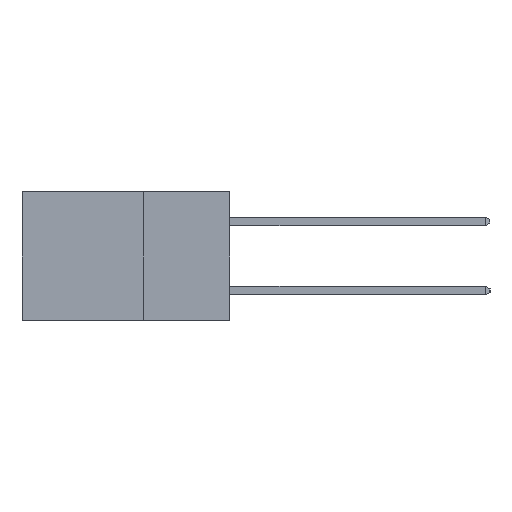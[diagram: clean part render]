
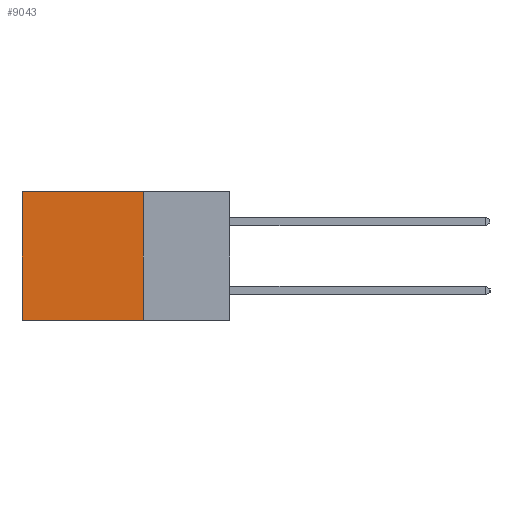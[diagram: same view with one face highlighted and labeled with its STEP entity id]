
A CAD part, left-side view. The second image highlights one B-rep face of the part: STEP entity #9043.
In plain terms, the highlighted planar face has unit normal (-1, 0, 0).
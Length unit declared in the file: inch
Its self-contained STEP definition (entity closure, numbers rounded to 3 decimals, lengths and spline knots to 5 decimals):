
#22 = CARTESIAN_POINT ( 'NONE',  ( 0.2615, 0.25, 0. ) ) ;
#853 = ORIENTED_EDGE ( 'NONE', *, *, #17617, .F. ) ;
#1217 = LINE ( 'NONE', #5633, #9360 ) ;
#1720 = ORIENTED_EDGE ( 'NONE', *, *, #5331, .T. ) ;
#2289 = EDGE_CURVE ( 'NONE', #4972, #5631, #1217, .T. ) ;
#2416 = CARTESIAN_POINT ( 'NONE',  ( 0.2615, 0.25, -0.37 ) ) ;
#2460 = FACE_OUTER_BOUND ( 'NONE', #6613, .T. ) ;
#3838 = VECTOR ( 'NONE', #12416, 39.37008 ) ;
#4061 = DIRECTION ( 'NONE',  ( 0., 0., -1. ) ) ;
#4581 = CARTESIAN_POINT ( 'NONE',  ( 0.2615, 0.6, 0. ) ) ;
#4972 = VERTEX_POINT ( 'NONE', #22 ) ;
#5236 = VERTEX_POINT ( 'NONE', #17708 ) ;
#5331 = EDGE_CURVE ( 'NONE', #5631, #5236, #5470, .T. ) ;
#5470 = LINE ( 'NONE', #16130, #13399 ) ;
#5631 = VERTEX_POINT ( 'NONE', #4581 ) ;
#5633 = CARTESIAN_POINT ( 'NONE',  ( 0.2615, 0.25, 0. ) ) ;
#6613 = EDGE_LOOP ( 'NONE', ( #1720, #853, #10607, #8937 ) ) ;
#7874 = VECTOR ( 'NONE', #10093, 39.37008 ) ;
#8937 = ORIENTED_EDGE ( 'NONE', *, *, #2289, .T. ) ;
#9043 = ADVANCED_FACE ( 'NONE', ( #2460 ), #12059, .F. ) ;
#9360 = VECTOR ( 'NONE', #15056, 39.37008 ) ;
#10093 = DIRECTION ( 'NONE',  ( 0., 1., 0. ) ) ;
#10607 = ORIENTED_EDGE ( 'NONE', *, *, #16162, .F. ) ;
#10828 = CARTESIAN_POINT ( 'NONE',  ( 0.2615, 0.25, -0.37 ) ) ;
#11309 = VERTEX_POINT ( 'NONE', #18542 ) ;
#11582 = CARTESIAN_POINT ( 'NONE',  ( 0.2615, 0.25, -0.37 ) ) ;
#12059 = PLANE ( 'NONE',  #14139 ) ;
#12416 = DIRECTION ( 'NONE',  ( 0., 0., -1. ) ) ;
#13399 = VECTOR ( 'NONE', #16199, 39.37008 ) ;
#13585 = DIRECTION ( 'NONE',  ( 1., 0., 0. ) ) ;
#14139 = AXIS2_PLACEMENT_3D ( 'NONE', #2416, #13585, #4061 ) ;
#15056 = DIRECTION ( 'NONE',  ( 0., 1., 0. ) ) ;
#16130 = CARTESIAN_POINT ( 'NONE',  ( 0.2615, 0.6, -0.37 ) ) ;
#16162 = EDGE_CURVE ( 'NONE', #4972, #11309, #16332, .T. ) ;
#16199 = DIRECTION ( 'NONE',  ( 0., 0., -1. ) ) ;
#16332 = LINE ( 'NONE', #10828, #3838 ) ;
#17617 = EDGE_CURVE ( 'NONE', #11309, #5236, #19938, .T. ) ;
#17708 = CARTESIAN_POINT ( 'NONE',  ( 0.2615, 0.6, -0.37 ) ) ;
#18542 = CARTESIAN_POINT ( 'NONE',  ( 0.2615, 0.25, -0.37 ) ) ;
#19938 = LINE ( 'NONE', #11582, #7874 ) ;
